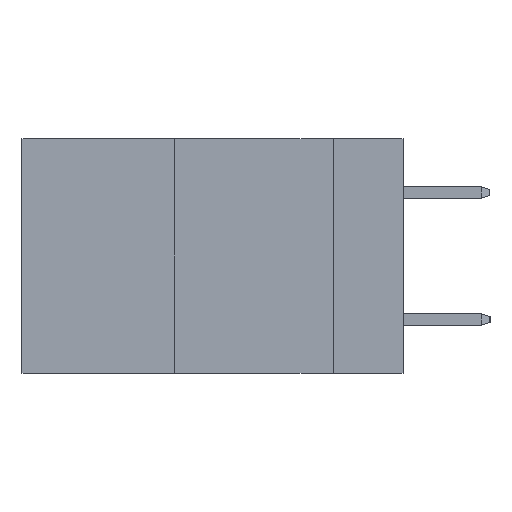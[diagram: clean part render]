
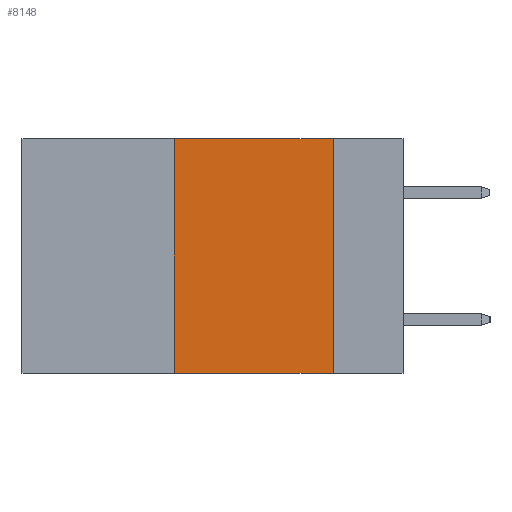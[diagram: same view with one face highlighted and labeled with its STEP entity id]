
A CAD part, left-side view. The second image highlights one B-rep face of the part: STEP entity #8148.
In plain terms, the highlighted planar face has unit normal (-1, 0, 0).
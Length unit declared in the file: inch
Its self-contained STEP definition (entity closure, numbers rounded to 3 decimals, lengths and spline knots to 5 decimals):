
#427 = VERTEX_POINT ( 'NONE', #740 ) ;
#518 = PLANE ( 'NONE',  #5053 ) ;
#740 = CARTESIAN_POINT ( 'NONE',  ( 0., 0.11, 0. ) ) ;
#1345 = DIRECTION ( 'NONE',  ( 0., 0., -1. ) ) ;
#1355 = ORIENTED_EDGE ( 'NONE', *, *, #7490, .F. ) ;
#1395 = LINE ( 'NONE', #1553, #8652 ) ;
#1502 = EDGE_CURVE ( 'NONE', #3655, #427, #8408, .T. ) ;
#1553 = CARTESIAN_POINT ( 'NONE',  ( 0., 0.36, 0. ) ) ;
#2022 = ORIENTED_EDGE ( 'NONE', *, *, #1502, .F. ) ;
#2325 = CARTESIAN_POINT ( 'NONE',  ( 0., 0.6, 0. ) ) ;
#2447 = CARTESIAN_POINT ( 'NONE',  ( 0., 0.36, 0. ) ) ;
#2946 = VERTEX_POINT ( 'NONE', #7514 ) ;
#3127 = CARTESIAN_POINT ( 'NONE',  ( 0., 0.11, 0. ) ) ;
#3655 = VERTEX_POINT ( 'NONE', #2447 ) ;
#4049 = DIRECTION ( 'NONE',  ( 0., -1., 0. ) ) ;
#4782 = VERTEX_POINT ( 'NONE', #5092 ) ;
#5053 = AXIS2_PLACEMENT_3D ( 'NONE', #2325, #9884, #7289 ) ;
#5066 = CARTESIAN_POINT ( 'NONE',  ( 0., 0.6, 0. ) ) ;
#5092 = CARTESIAN_POINT ( 'NONE',  ( 0., 0.36, -0.37 ) ) ;
#5745 = VECTOR ( 'NONE', #9796, 39.37008 ) ;
#5859 = VECTOR ( 'NONE', #4049, 39.37008 ) ;
#6269 = EDGE_LOOP ( 'NONE', ( #1355, #2022, #9003, #7090 ) ) ;
#6856 = EDGE_CURVE ( 'NONE', #4782, #2946, #8884, .T. ) ;
#7003 = VECTOR ( 'NONE', #1345, 39.37008 ) ;
#7090 = ORIENTED_EDGE ( 'NONE', *, *, #6856, .T. ) ;
#7289 = DIRECTION ( 'NONE',  ( 0., 0., -1. ) ) ;
#7490 = EDGE_CURVE ( 'NONE', #427, #2946, #8917, .T. ) ;
#7514 = CARTESIAN_POINT ( 'NONE',  ( 0., 0.11, -0.37 ) ) ;
#8148 = ADVANCED_FACE ( 'NONE', ( #9774 ), #518, .F. ) ;
#8408 = LINE ( 'NONE', #5066, #5859 ) ;
#8652 = VECTOR ( 'NONE', #9875, 39.37008 ) ;
#8884 = LINE ( 'NONE', #10681, #5745 ) ;
#8917 = LINE ( 'NONE', #3127, #7003 ) ;
#9003 = ORIENTED_EDGE ( 'NONE', *, *, #9906, .F. ) ;
#9774 = FACE_OUTER_BOUND ( 'NONE', #6269, .T. ) ;
#9796 = DIRECTION ( 'NONE',  ( 0., -1., 0. ) ) ;
#9875 = DIRECTION ( 'NONE',  ( 0., 0., 1. ) ) ;
#9884 = DIRECTION ( 'NONE',  ( 1., 0., 0. ) ) ;
#9906 = EDGE_CURVE ( 'NONE', #4782, #3655, #1395, .T. ) ;
#10681 = CARTESIAN_POINT ( 'NONE',  ( 0., 0.6, -0.37 ) ) ;
